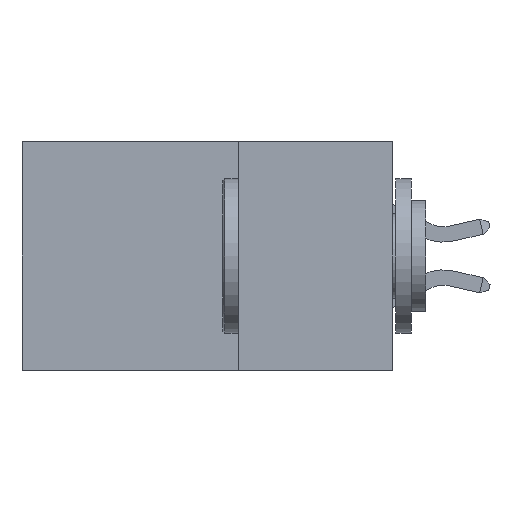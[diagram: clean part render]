
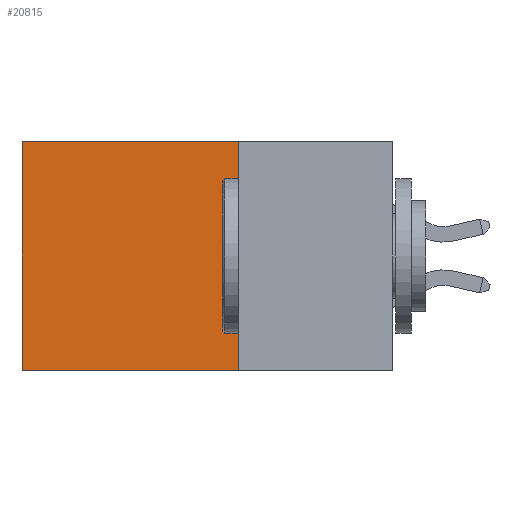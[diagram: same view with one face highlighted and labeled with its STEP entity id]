
A CAD part, left-side view. The second image highlights one B-rep face of the part: STEP entity #20815.
In plain terms, the highlighted planar face has unit normal (-1, 0, 0).
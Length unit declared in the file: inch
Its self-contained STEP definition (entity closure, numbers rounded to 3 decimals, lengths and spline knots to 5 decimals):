
#643 = DIRECTION ( 'NONE',  ( 1., 0., 0. ) ) ;
#926 = VECTOR ( 'NONE', #20752, 39.37008 ) ;
#1681 = ORIENTED_EDGE ( 'NONE', *, *, #25150, .T. ) ;
#2830 = CARTESIAN_POINT ( 'NONE',  ( 0.2875, 0.6, 0. ) ) ;
#3349 = LINE ( 'NONE', #9740, #26209 ) ;
#3928 = EDGE_CURVE ( 'NONE', #13023, #11685, #3349, .T. ) ;
#4600 = ORIENTED_EDGE ( 'NONE', *, *, #3928, .F. ) ;
#6788 = VERTEX_POINT ( 'NONE', #16497 ) ;
#7062 = DIRECTION ( 'NONE',  ( 0., 0., -1. ) ) ;
#8180 = EDGE_LOOP ( 'NONE', ( #1681, #4600, #22725, #8598 ) ) ;
#8492 = VERTEX_POINT ( 'NONE', #19794 ) ;
#8598 = ORIENTED_EDGE ( 'NONE', *, *, #28586, .T. ) ;
#8727 = PLANE ( 'NONE',  #20598 ) ;
#9562 = CARTESIAN_POINT ( 'NONE',  ( 0.2875, 0.6, -0.37 ) ) ;
#9740 = CARTESIAN_POINT ( 'NONE',  ( 0.2875, 0.25, -0.37 ) ) ;
#11685 = VERTEX_POINT ( 'NONE', #9562 ) ;
#11976 = DIRECTION ( 'NONE',  ( 0., 1., 0. ) ) ;
#12881 = VECTOR ( 'NONE', #15902, 39.37008 ) ;
#13023 = VERTEX_POINT ( 'NONE', #27451 ) ;
#15814 = CARTESIAN_POINT ( 'NONE',  ( 0.2875, 0.25, 0. ) ) ;
#15902 = DIRECTION ( 'NONE',  ( 0., 0., -1. ) ) ;
#16495 = DIRECTION ( 'NONE',  ( 0., 0., -1. ) ) ;
#16497 = CARTESIAN_POINT ( 'NONE',  ( 0.2875, 0.6, 0. ) ) ;
#18498 = EDGE_CURVE ( 'NONE', #8492, #13023, #26629, .T. ) ;
#18625 = CARTESIAN_POINT ( 'NONE',  ( 0.2875, 0.25, 0. ) ) ;
#19794 = CARTESIAN_POINT ( 'NONE',  ( 0.2875, 0.25, 0. ) ) ;
#20188 = CARTESIAN_POINT ( 'NONE',  ( 0.2875, 0.25, 0. ) ) ;
#20598 = AXIS2_PLACEMENT_3D ( 'NONE', #20188, #643, #16495 ) ;
#20752 = DIRECTION ( 'NONE',  ( 0., 1., 0. ) ) ;
#20815 = ADVANCED_FACE ( 'NONE', ( #22350 ), #8727, .F. ) ;
#20998 = LINE ( 'NONE', #18625, #926 ) ;
#22350 = FACE_OUTER_BOUND ( 'NONE', #8180, .T. ) ;
#22725 = ORIENTED_EDGE ( 'NONE', *, *, #18498, .F. ) ;
#22927 = LINE ( 'NONE', #2830, #12881 ) ;
#23857 = VECTOR ( 'NONE', #7062, 39.37008 ) ;
#25150 = EDGE_CURVE ( 'NONE', #6788, #11685, #22927, .T. ) ;
#26209 = VECTOR ( 'NONE', #11976, 39.37008 ) ;
#26629 = LINE ( 'NONE', #15814, #23857 ) ;
#27451 = CARTESIAN_POINT ( 'NONE',  ( 0.2875, 0.25, -0.37 ) ) ;
#28586 = EDGE_CURVE ( 'NONE', #8492, #6788, #20998, .T. ) ;
